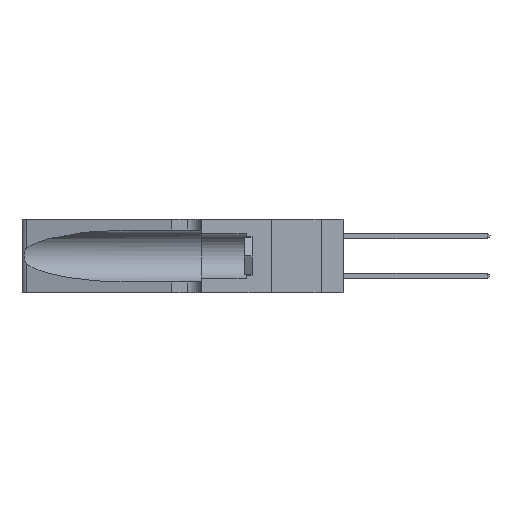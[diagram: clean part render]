
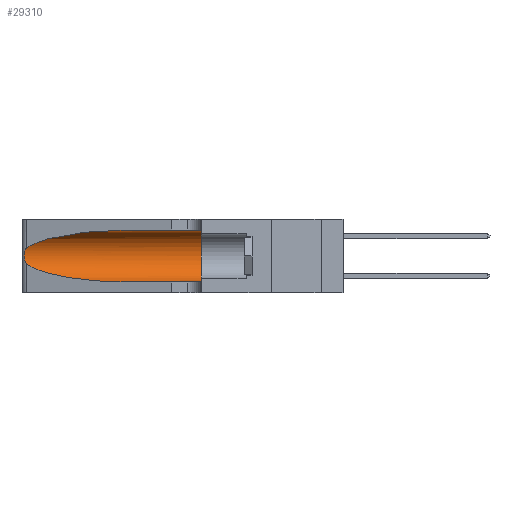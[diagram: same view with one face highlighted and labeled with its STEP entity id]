
A CAD part, left-side view. The second image highlights one B-rep face of the part: STEP entity #29310.
In plain terms, the highlighted cylindrical face has radius 3.308 mm (diameter 6.617 mm), a partial arc.
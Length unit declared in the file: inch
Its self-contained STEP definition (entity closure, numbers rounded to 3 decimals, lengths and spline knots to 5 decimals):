
#220 = CARTESIAN_POINT ( 'NONE',  ( 0.1305, 1.61858, 0.31525 ) ) ;
#434 = DIRECTION ( 'NONE',  ( 0., 0., -1. ) ) ;
#844 = ORIENTED_EDGE ( 'NONE', *, *, #35059, .F. ) ;
#1165 = CYLINDRICAL_SURFACE ( 'NONE', #34729, 0.13025 ) ;
#1617 = VECTOR ( 'NONE', #41657, 39.37008 ) ;
#1984 = CARTESIAN_POINT ( 'NONE',  ( 0.2373, 1.15595, 0.28018 ) ) ;
#2167 = VERTEX_POINT ( 'NONE', #35815 ) ;
#2755 = ORIENTED_EDGE ( 'NONE', *, *, #15539, .F. ) ;
#4176 = CARTESIAN_POINT ( 'NONE',  ( 0.25789, 1.23486, 0.15765 ) ) ;
#6989 = CARTESIAN_POINT ( 'NONE',  ( 0.25787, 1.23484, 0.2124 ) ) ;
#7304 = CARTESIAN_POINT ( 'NONE',  ( 0.25639, 1.23186, 0.15144 ) ) ;
#7787 = CARTESIAN_POINT ( 'NONE',  ( 0.26017, 1.23833, 0.17102 ) ) ;
#7882 = AXIS2_PLACEMENT_3D ( 'NONE', #11786, #11628, #22138 ) ;
#7883 = CARTESIAN_POINT ( 'NONE',  ( 0.25487, 1.22718, 0.22369 ) ) ;
#10449 = CARTESIAN_POINT ( 'NONE',  ( 0.25487, 1.22718, 0.22369 ) ) ;
#10937 = ORIENTED_EDGE ( 'NONE', *, *, #11118, .T. ) ;
#11118 = EDGE_CURVE ( 'NONE', #29158, #23238, #29515, .T. ) ;
#11628 = DIRECTION ( 'NONE',  ( 0., 1., 0. ) ) ;
#11786 = CARTESIAN_POINT ( 'NONE',  ( 0.1305, 0.35, 0.185 ) ) ;
#12400 = ORIENTED_EDGE ( 'NONE', *, *, #45835, .T. ) ;
#13995 = CARTESIAN_POINT ( 'NONE',  ( 0.25854, 1.2359, 0.20912 ) ) ;
#15539 = EDGE_CURVE ( 'NONE', #2167, #45515, #22315, .T. ) ;
#16007 = CARTESIAN_POINT ( 'NONE',  ( 0.18966, 0.96281, 0.31525 ) ) ;
#17729 = CARTESIAN_POINT ( 'NONE',  ( 0.2373, 1.15595, 0.08982 ) ) ;
#18033 = CARTESIAN_POINT ( 'NONE',  ( 0.25487, 1.22718, 0.14631 ) ) ;
#20989 = CARTESIAN_POINT ( 'NONE',  ( 0.1305, 0.72297, 0.31525 ) ) ;
#21584 = CARTESIAN_POINT ( 'NONE',  ( 0.1305, 0.72297, 0.05475 ) ) ;
#22138 = DIRECTION ( 'NONE',  ( 0., 0., 1. ) ) ;
#22315 = CIRCLE ( 'NONE', #7882, 0.13025 ) ;
#22897 = VERTEX_POINT ( 'NONE', #42272 ) ;
#22996 = ORIENTED_EDGE ( 'NONE', *, *, #29093, .T. ) ;
#23238 = VERTEX_POINT ( 'NONE', #7883 ) ;
#24676 = CARTESIAN_POINT ( 'NONE',  ( 0.26075, 1.23896, 0.19203 ) ) ;
#24987 = CARTESIAN_POINT ( 'NONE',  ( 0.25856, 1.23593, 0.16098 ) ) ;
#25484 = CARTESIAN_POINT ( 'NONE',  ( 0.1305, 0.35, 0.05475 ) ) ;
#26380 = CARTESIAN_POINT ( 'NONE',  ( 0.25487, 1.22718, 0.22369 ) ) ;
#27059 = VERTEX_POINT ( 'NONE', #44426 ) ;
#28251 = CARTESIAN_POINT ( 'NONE',  ( 0.26075, 1.23896, 0.178 ) ) ;
#28341 =( BOUNDED_CURVE ( )  B_SPLINE_CURVE ( 3, ( #18033, #17729, #38910, #21584 ),
 .UNSPECIFIED., .F., .F. ) 
 B_SPLINE_CURVE_WITH_KNOTS ( ( 4, 4 ),
 ( 3.44316, 4.71239 ),
 .UNSPECIFIED. ) 
 CURVE ( )  GEOMETRIC_REPRESENTATION_ITEM ( )  RATIONAL_B_SPLINE_CURVE ( ( 1., 0.87, 0.87, 1. ) ) 
 REPRESENTATION_ITEM ( '' )  );
#29093 = EDGE_CURVE ( 'NONE', #27059, #22897, #28341, .T. ) ;
#29158 = VERTEX_POINT ( 'NONE', #20989 ) ;
#29310 = ADVANCED_FACE ( 'NONE', ( #39580 ), #1165, .F. ) ;
#29515 =( BOUNDED_CURVE ( )  B_SPLINE_CURVE ( 3, ( #37615, #16007, #1984, #26380 ),
 .UNSPECIFIED., .F., .F. ) 
 B_SPLINE_CURVE_WITH_KNOTS ( ( 4, 4 ),
 ( 1.5708, 2.84003 ),
 .UNSPECIFIED. ) 
 CURVE ( )  GEOMETRIC_REPRESENTATION_ITEM ( )  RATIONAL_B_SPLINE_CURVE ( ( 1., 0.87, 0.87, 1. ) ) 
 REPRESENTATION_ITEM ( '' )  );
#30055 = EDGE_CURVE ( 'NONE', #22897, #45515, #33355, .T. ) ;
#32266 = DIRECTION ( 'NONE',  ( 0., -1., 0. ) ) ;
#33355 = LINE ( 'NONE', #38202, #1617 ) ;
#34195 = VECTOR ( 'NONE', #32266, 39.37008 ) ;
#34729 = AXIS2_PLACEMENT_3D ( 'NONE', #40016, #43740, #434 ) ;
#35059 = EDGE_CURVE ( 'NONE', #29158, #2167, #37557, .T. ) ;
#35277 = CARTESIAN_POINT ( 'NONE',  ( 0.25555, 1.22994, 0.2215 ) ) ;
#35815 = CARTESIAN_POINT ( 'NONE',  ( 0.1305, 0.35, 0.31525 ) ) ;
#36065 = B_SPLINE_CURVE_WITH_KNOTS ( 'NONE', 3,
 ( #10449, #35277, #46042, #6989, #13995, #38875, #24676, #28251, #7787, #24987, #4176, #7304, #42922, #39497 ),
 .UNSPECIFIED., .F., .F.,
 ( 4, 2, 2, 2, 2, 2, 4 ),
 ( 0., 0.00027, 0.00053, 0.00107, 0.0016, 0.00187, 0.00214 ),
 .UNSPECIFIED. ) ;
#37557 = LINE ( 'NONE', #220, #34195 ) ;
#37615 = CARTESIAN_POINT ( 'NONE',  ( 0.1305, 0.72297, 0.31525 ) ) ;
#38202 = CARTESIAN_POINT ( 'NONE',  ( 0.1305, 1.61858, 0.05475 ) ) ;
#38875 = CARTESIAN_POINT ( 'NONE',  ( 0.26018, 1.23835, 0.19895 ) ) ;
#38910 = CARTESIAN_POINT ( 'NONE',  ( 0.18966, 0.96281, 0.05475 ) ) ;
#39206 = EDGE_LOOP ( 'NONE', ( #10937, #12400, #22996, #43230, #2755, #844 ) ) ;
#39497 = CARTESIAN_POINT ( 'NONE',  ( 0.25487, 1.22718, 0.14631 ) ) ;
#39580 = FACE_OUTER_BOUND ( 'NONE', #39206, .T. ) ;
#40016 = CARTESIAN_POINT ( 'NONE',  ( 0.1305, 1.61858, 0.185 ) ) ;
#41657 = DIRECTION ( 'NONE',  ( 0., -1., 0. ) ) ;
#42272 = CARTESIAN_POINT ( 'NONE',  ( 0.1305, 0.72297, 0.05475 ) ) ;
#42922 = CARTESIAN_POINT ( 'NONE',  ( 0.25555, 1.22993, 0.14849 ) ) ;
#43230 = ORIENTED_EDGE ( 'NONE', *, *, #30055, .T. ) ;
#43740 = DIRECTION ( 'NONE',  ( 0., -1., 0. ) ) ;
#44426 = CARTESIAN_POINT ( 'NONE',  ( 0.25487, 1.22718, 0.14631 ) ) ;
#45515 = VERTEX_POINT ( 'NONE', #25484 ) ;
#45835 = EDGE_CURVE ( 'NONE', #23238, #27059, #36065, .T. ) ;
#46042 = CARTESIAN_POINT ( 'NONE',  ( 0.25639, 1.23184, 0.21858 ) ) ;
